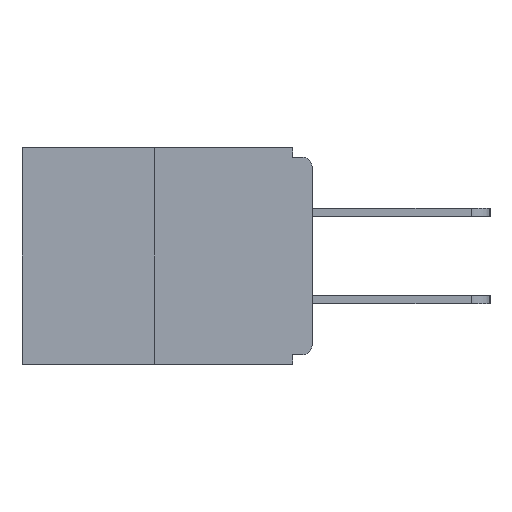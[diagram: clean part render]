
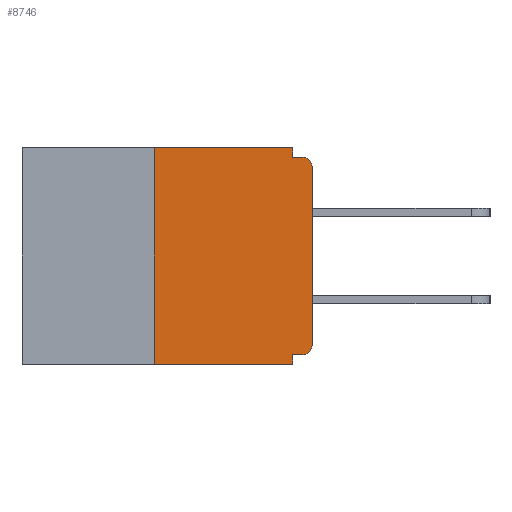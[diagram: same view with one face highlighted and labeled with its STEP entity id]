
A CAD part, left-side view. The second image highlights one B-rep face of the part: STEP entity #8746.
In plain terms, the highlighted planar face has unit normal (-1, 0, 0).
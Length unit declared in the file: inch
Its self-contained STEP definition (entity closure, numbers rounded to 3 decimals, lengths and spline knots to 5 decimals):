
#436 = VECTOR ( 'NONE', #6981, 39.37008 ) ;
#446 = LINE ( 'NONE', #10068, #6178 ) ;
#498 = ORIENTED_EDGE ( 'NONE', *, *, #10277, .F. ) ;
#534 = VECTOR ( 'NONE', #778, 39.37008 ) ;
#579 = DIRECTION ( 'NONE',  ( 1., 0., 0. ) ) ;
#649 = ORIENTED_EDGE ( 'NONE', *, *, #1639, .F. ) ;
#761 = VERTEX_POINT ( 'NONE', #8805 ) ;
#778 = DIRECTION ( 'NONE',  ( 0., -1., 0. ) ) ;
#809 = DIRECTION ( 'NONE',  ( 0., 1., 0. ) ) ;
#974 = EDGE_CURVE ( 'NONE', #12584, #3538, #8904, .T. ) ;
#1182 = DIRECTION ( 'NONE',  ( -1., 0., 0. ) ) ;
#1366 = CARTESIAN_POINT ( 'NONE',  ( 0., 0., -0.03 ) ) ;
#1639 = EDGE_CURVE ( 'NONE', #761, #7135, #446, .T. ) ;
#1714 = LINE ( 'NONE', #12117, #436 ) ;
#1775 = VERTEX_POINT ( 'NONE', #10962 ) ;
#1789 = ORIENTED_EDGE ( 'NONE', *, *, #7275, .T. ) ;
#2161 = VERTEX_POINT ( 'NONE', #12026 ) ;
#2168 = EDGE_CURVE ( 'NONE', #2194, #12584, #1714, .T. ) ;
#2194 = VERTEX_POINT ( 'NONE', #10061 ) ;
#2250 = DIRECTION ( 'NONE',  ( 0., 0., 1. ) ) ;
#2304 = CARTESIAN_POINT ( 'NONE',  ( 0., 0.015, -0.328 ) ) ;
#2575 = EDGE_CURVE ( 'NONE', #7729, #2161, #5330, .T. ) ;
#2596 = LINE ( 'NONE', #6449, #12996 ) ;
#2860 = DIRECTION ( 'NONE',  ( 0., -1., 0. ) ) ;
#2988 = VERTEX_POINT ( 'NONE', #1366 ) ;
#3049 = VECTOR ( 'NONE', #2250, 39.37008 ) ;
#3538 = VERTEX_POINT ( 'NONE', #6717 ) ;
#3554 = PLANE ( 'NONE',  #11727 ) ;
#3895 = CARTESIAN_POINT ( 'NONE',  ( 0., 0.46, -0.343 ) ) ;
#4034 = FACE_OUTER_BOUND ( 'NONE', #5555, .T. ) ;
#4523 = AXIS2_PLACEMENT_3D ( 'NONE', #11206, #7109, #10134 ) ;
#4748 = ORIENTED_EDGE ( 'NONE', *, *, #2575, .T. ) ;
#5330 = CIRCLE ( 'NONE', #11074, 0.015 ) ;
#5555 = EDGE_LOOP ( 'NONE', ( #9434, #9396, #7954, #6932, #8779, #4748, #5718, #1789, #649, #498 ) ) ;
#5718 = ORIENTED_EDGE ( 'NONE', *, *, #6759, .T. ) ;
#5750 = VECTOR ( 'NONE', #809, 39.37008 ) ;
#5763 = DIRECTION ( 'NONE',  ( 0., 0., -1. ) ) ;
#5992 = DIRECTION ( 'NONE',  ( 0., 0., -1. ) ) ;
#6178 = VECTOR ( 'NONE', #11319, 39.37008 ) ;
#6449 = CARTESIAN_POINT ( 'NONE',  ( 0., 0.031, -0.343 ) ) ;
#6509 = CIRCLE ( 'NONE', #4523, 0.015 ) ;
#6717 = CARTESIAN_POINT ( 'NONE',  ( 0., 0.031, 0. ) ) ;
#6759 = EDGE_CURVE ( 'NONE', #2161, #2988, #12328, .T. ) ;
#6858 = CARTESIAN_POINT ( 'NONE',  ( 0., 0., -0.328 ) ) ;
#6906 = VECTOR ( 'NONE', #2860, 39.37008 ) ;
#6932 = ORIENTED_EDGE ( 'NONE', *, *, #10582, .F. ) ;
#6981 = DIRECTION ( 'NONE',  ( 0., 0., 1. ) ) ;
#7109 = DIRECTION ( 'NONE',  ( -1., 0., 0. ) ) ;
#7135 = VERTEX_POINT ( 'NONE', #8542 ) ;
#7275 = EDGE_CURVE ( 'NONE', #2988, #7135, #6509, .T. ) ;
#7300 = CARTESIAN_POINT ( 'NONE',  ( 0., 0., 0. ) ) ;
#7729 = VERTEX_POINT ( 'NONE', #2304 ) ;
#7954 = ORIENTED_EDGE ( 'NONE', *, *, #8807, .T. ) ;
#8542 = CARTESIAN_POINT ( 'NONE',  ( 0., 0.015, -0.015 ) ) ;
#8746 = ADVANCED_FACE ( 'NONE', ( #4034 ), #3554, .F. ) ;
#8779 = ORIENTED_EDGE ( 'NONE', *, *, #10118, .F. ) ;
#8805 = CARTESIAN_POINT ( 'NONE',  ( 0., 0.031, -0.015 ) ) ;
#8807 = EDGE_CURVE ( 'NONE', #2194, #1775, #10216, .T. ) ;
#8904 = LINE ( 'NONE', #10768, #534 ) ;
#8922 = CARTESIAN_POINT ( 'NONE',  ( 0., 0.031, 0. ) ) ;
#9195 = VECTOR ( 'NONE', #5992, 39.37008 ) ;
#9196 = CARTESIAN_POINT ( 'NONE',  ( 0., 0.031, -0.328 ) ) ;
#9295 = DIRECTION ( 'NONE',  ( 0., 0., -1. ) ) ;
#9396 = ORIENTED_EDGE ( 'NONE', *, *, #2168, .F. ) ;
#9434 = ORIENTED_EDGE ( 'NONE', *, *, #974, .F. ) ;
#9521 = LINE ( 'NONE', #6858, #5750 ) ;
#9788 = CARTESIAN_POINT ( 'NONE',  ( 0., 0.46, 0. ) ) ;
#10061 = CARTESIAN_POINT ( 'NONE',  ( 0., 0.25, -0.343 ) ) ;
#10068 = CARTESIAN_POINT ( 'NONE',  ( 0., 0., -0.015 ) ) ;
#10118 = EDGE_CURVE ( 'NONE', #7729, #12520, #9521, .T. ) ;
#10134 = DIRECTION ( 'NONE',  ( 0., 0., -1. ) ) ;
#10216 = LINE ( 'NONE', #3895, #6906 ) ;
#10277 = EDGE_CURVE ( 'NONE', #3538, #761, #10795, .T. ) ;
#10326 = DIRECTION ( 'NONE',  ( 0., 0., -1. ) ) ;
#10582 = EDGE_CURVE ( 'NONE', #12520, #1775, #2596, .T. ) ;
#10608 = CARTESIAN_POINT ( 'NONE',  ( 0., 0.25, 0. ) ) ;
#10768 = CARTESIAN_POINT ( 'NONE',  ( 0., 0.46, 0. ) ) ;
#10795 = LINE ( 'NONE', #8922, #9195 ) ;
#10962 = CARTESIAN_POINT ( 'NONE',  ( 0., 0.031, -0.343 ) ) ;
#11074 = AXIS2_PLACEMENT_3D ( 'NONE', #11292, #1182, #9295 ) ;
#11206 = CARTESIAN_POINT ( 'NONE',  ( 0., 0.015, -0.03 ) ) ;
#11292 = CARTESIAN_POINT ( 'NONE',  ( 0., 0.015, -0.313 ) ) ;
#11319 = DIRECTION ( 'NONE',  ( 0., -1., 0. ) ) ;
#11727 = AXIS2_PLACEMENT_3D ( 'NONE', #9788, #579, #5763 ) ;
#12026 = CARTESIAN_POINT ( 'NONE',  ( 0., 0., -0.313 ) ) ;
#12117 = CARTESIAN_POINT ( 'NONE',  ( 0., 0.25, 0. ) ) ;
#12328 = LINE ( 'NONE', #7300, #3049 ) ;
#12520 = VERTEX_POINT ( 'NONE', #9196 ) ;
#12584 = VERTEX_POINT ( 'NONE', #10608 ) ;
#12996 = VECTOR ( 'NONE', #10326, 39.37008 ) ;
